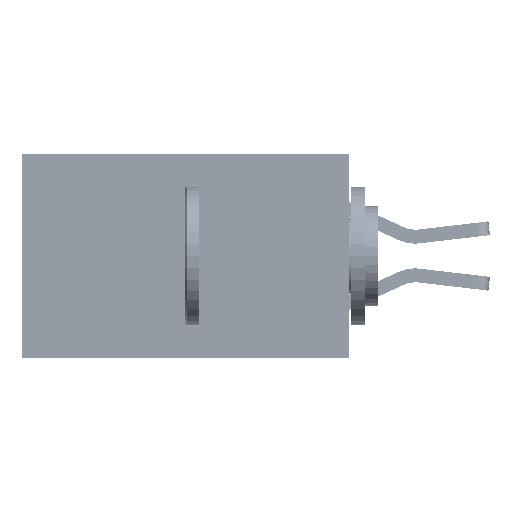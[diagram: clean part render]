
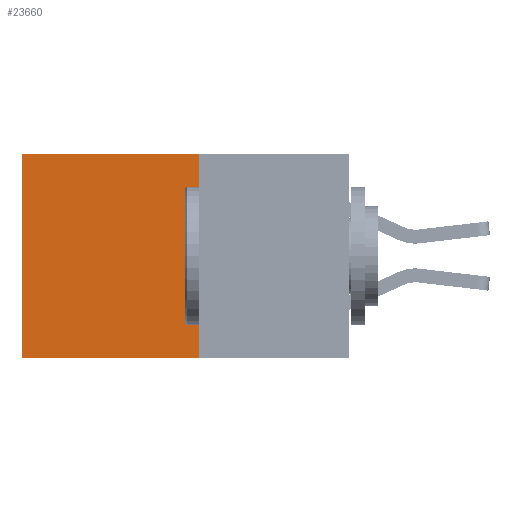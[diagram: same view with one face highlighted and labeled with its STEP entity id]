
A CAD part, left-side view. The second image highlights one B-rep face of the part: STEP entity #23660.
In plain terms, the highlighted planar face has unit normal (-1, 0, 0).
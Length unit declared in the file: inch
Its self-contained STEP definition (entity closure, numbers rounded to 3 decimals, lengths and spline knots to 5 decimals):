
#730 = CARTESIAN_POINT ( 'NONE',  ( 0.277, 0.59, -0.37 ) ) ;
#5515 = ORIENTED_EDGE ( 'NONE', *, *, #16962, .F. ) ;
#6226 = DIRECTION ( 'NONE',  ( 0., 0., -1. ) ) ;
#6745 = ORIENTED_EDGE ( 'NONE', *, *, #16072, .T. ) ;
#7322 = FACE_OUTER_BOUND ( 'NONE', #13582, .T. ) ;
#7606 = CARTESIAN_POINT ( 'NONE',  ( 0.277, 0.27, -0.37 ) ) ;
#8698 = LINE ( 'NONE', #27163, #21105 ) ;
#8730 = CARTESIAN_POINT ( 'NONE',  ( 0.277, 0.59, -0.37 ) ) ;
#8967 = CARTESIAN_POINT ( 'NONE',  ( 0.277, 0.27, -0.37 ) ) ;
#9112 = VERTEX_POINT ( 'NONE', #20241 ) ;
#9211 = VECTOR ( 'NONE', #15033, 39.37008 ) ;
#9973 = LINE ( 'NONE', #27396, #9211 ) ;
#10287 = LINE ( 'NONE', #8730, #21931 ) ;
#10313 = EDGE_CURVE ( 'NONE', #11601, #20494, #25276, .T. ) ;
#11424 = DIRECTION ( 'NONE',  ( 0., 0., -1. ) ) ;
#11601 = VERTEX_POINT ( 'NONE', #14528 ) ;
#12661 = DIRECTION ( 'NONE',  ( 0., 0., -1. ) ) ;
#13065 = ORIENTED_EDGE ( 'NONE', *, *, #14916, .T. ) ;
#13582 = EDGE_LOOP ( 'NONE', ( #6745, #5515, #23376, #13065 ) ) ;
#14528 = CARTESIAN_POINT ( 'NONE',  ( 0.277, 0.27, 0. ) ) ;
#14916 = EDGE_CURVE ( 'NONE', #11601, #9112, #9973, .T. ) ;
#15033 = DIRECTION ( 'NONE',  ( 0., 1., 0. ) ) ;
#16072 = EDGE_CURVE ( 'NONE', #9112, #30169, #10287, .T. ) ;
#16962 = EDGE_CURVE ( 'NONE', #20494, #30169, #8698, .T. ) ;
#17384 = AXIS2_PLACEMENT_3D ( 'NONE', #8967, #26266, #11424 ) ;
#20241 = CARTESIAN_POINT ( 'NONE',  ( 0.277, 0.59, 0. ) ) ;
#20494 = VERTEX_POINT ( 'NONE', #30085 ) ;
#21105 = VECTOR ( 'NONE', #29634, 39.37008 ) ;
#21321 = PLANE ( 'NONE',  #17384 ) ;
#21931 = VECTOR ( 'NONE', #6226, 39.37008 ) ;
#23376 = ORIENTED_EDGE ( 'NONE', *, *, #10313, .F. ) ;
#23660 = ADVANCED_FACE ( 'NONE', ( #7322 ), #21321, .F. ) ;
#25276 = LINE ( 'NONE', #7606, #31043 ) ;
#26266 = DIRECTION ( 'NONE',  ( 1., 0., 0. ) ) ;
#27163 = CARTESIAN_POINT ( 'NONE',  ( 0.277, 0.27, -0.37 ) ) ;
#27396 = CARTESIAN_POINT ( 'NONE',  ( 0.277, 0.27, 0. ) ) ;
#29634 = DIRECTION ( 'NONE',  ( 0., 1., 0. ) ) ;
#30085 = CARTESIAN_POINT ( 'NONE',  ( 0.277, 0.27, -0.37 ) ) ;
#30169 = VERTEX_POINT ( 'NONE', #730 ) ;
#31043 = VECTOR ( 'NONE', #12661, 39.37008 ) ;
